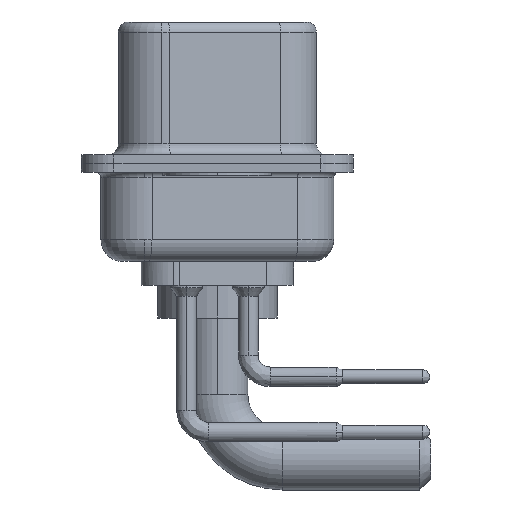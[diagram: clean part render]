
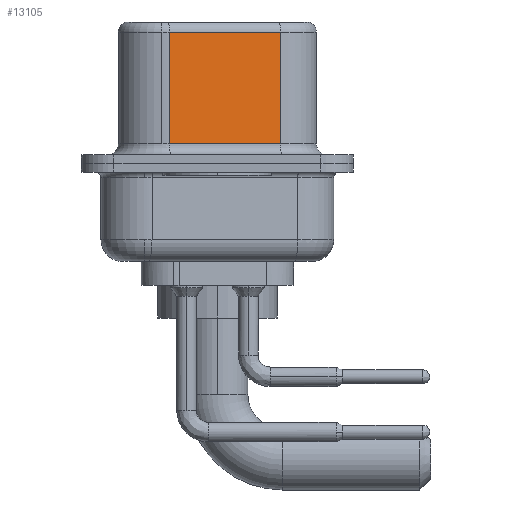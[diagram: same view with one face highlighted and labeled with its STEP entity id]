
A CAD part, left-side view. The second image highlights one B-rep face of the part: STEP entity #13105.
In plain terms, the highlighted planar face has unit normal (-0.985, -0.174, 0).
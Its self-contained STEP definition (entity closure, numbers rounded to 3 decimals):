
#75 = CARTESIAN_POINT ( 'NONE',  ( 4.555, -2.897, 0.9 ) ) ;
#400 = VERTEX_POINT ( 'NONE', #6358 ) ;
#828 = LINE ( 'NONE', #11886, #12910 ) ;
#979 = CARTESIAN_POINT ( 'NONE',  ( 4.555, -2.897, 6.02 ) ) ;
#1323 = ORIENTED_EDGE ( 'NONE', *, *, #10759, .T. ) ;
#1638 = LINE ( 'NONE', #75, #9240 ) ;
#1827 = ORIENTED_EDGE ( 'NONE', *, *, #16366, .T. ) ;
#2572 = VERTEX_POINT ( 'NONE', #8710 ) ;
#3496 = DIRECTION ( 'NONE',  ( 0.174, -0.985, 0. ) ) ;
#5172 = DIRECTION ( 'NONE',  ( 0., 0., -1. ) ) ;
#5659 = VECTOR ( 'NONE', #5172, 1000. ) ;
#6358 = CARTESIAN_POINT ( 'NONE',  ( 4.555, -2.897, 6.02 ) ) ;
#6653 = VERTEX_POINT ( 'NONE', #14393 ) ;
#6746 = LINE ( 'NONE', #9993, #5659 ) ;
#6867 = VECTOR ( 'NONE', #13693, 1000. ) ;
#7772 = EDGE_CURVE ( 'NONE', #400, #2572, #10378, .T. ) ;
#8057 = CARTESIAN_POINT ( 'NONE',  ( 3.655, 2.203, 0.9 ) ) ;
#8710 = CARTESIAN_POINT ( 'NONE',  ( 3.655, 2.203, 6.02 ) ) ;
#8919 = ORIENTED_EDGE ( 'NONE', *, *, #7772, .T. ) ;
#9196 = EDGE_LOOP ( 'NONE', ( #13517, #8919, #1323, #1827 ) ) ;
#9240 = VECTOR ( 'NONE', #3496, 1000. ) ;
#9848 = DIRECTION ( 'NONE',  ( 0.985, 0.174, 0. ) ) ;
#9993 = CARTESIAN_POINT ( 'NONE',  ( 4.555, -2.897, 6.52 ) ) ;
#10378 = LINE ( 'NONE', #979, #6867 ) ;
#10639 = DIRECTION ( 'NONE',  ( 0., 0., -1. ) ) ;
#10759 = EDGE_CURVE ( 'NONE', #2572, #18989, #828, .T. ) ;
#11412 = CARTESIAN_POINT ( 'NONE',  ( 4.555, -2.897, 6.52 ) ) ;
#11711 = DIRECTION ( 'NONE',  ( -0.174, 0.985, 0. ) ) ;
#11886 = CARTESIAN_POINT ( 'NONE',  ( 3.655, 2.203, 6.52 ) ) ;
#12910 = VECTOR ( 'NONE', #10639, 1000. ) ;
#12912 = EDGE_CURVE ( 'NONE', #400, #6653, #6746, .T. ) ;
#13105 = ADVANCED_FACE ( 'NONE', ( #19290 ), #19489, .F. ) ;
#13517 = ORIENTED_EDGE ( 'NONE', *, *, #12912, .F. ) ;
#13693 = DIRECTION ( 'NONE',  ( -0.174, 0.985, 0. ) ) ;
#14393 = CARTESIAN_POINT ( 'NONE',  ( 4.555, -2.897, 0.9 ) ) ;
#16366 = EDGE_CURVE ( 'NONE', #18989, #6653, #1638, .T. ) ;
#18970 = AXIS2_PLACEMENT_3D ( 'NONE', #11412, #9848, #11711 ) ;
#18989 = VERTEX_POINT ( 'NONE', #8057 ) ;
#19290 = FACE_OUTER_BOUND ( 'NONE', #9196, .T. ) ;
#19489 = PLANE ( 'NONE',  #18970 ) ;
